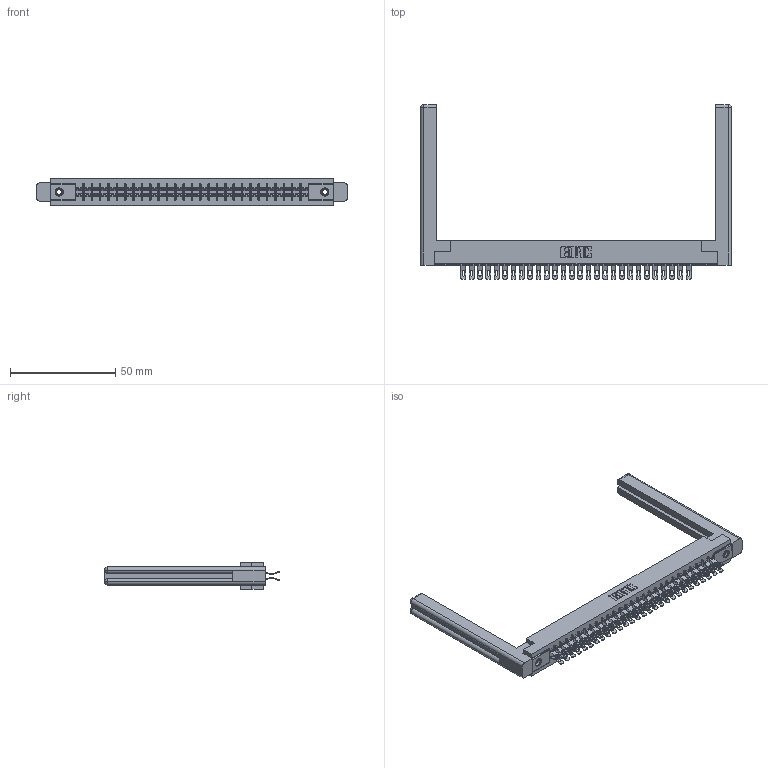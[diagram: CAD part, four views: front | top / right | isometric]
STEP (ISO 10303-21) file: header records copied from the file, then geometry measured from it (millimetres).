
FILE_DESCRIPTION (( 'STEP AP203' ), '1' );
FILE_NAME ('305-056-555-558.STEP', '2019-09-09T23:57:06', ( '' ), ( '' ), 'SwSTEP 2.0', 'SolidWorks 2016', '' );
FILE_SCHEMA (( 'CONFIG_CONTROL_DESIGN' ));
Length unit declared in the file: inch
Products named in the file (5): 305-056-555-558; 307-220-058; 305-290-001_555; 345-250-001_345-250-001-102; 305 Part_.156 Dia
Assembly tree (61 placements, depth 2):
  305-056-555-558
    305 Part_.156 Dia
    305-290-001_555  x56
    345-250-001_345-250-001-102  x2
    307-220-058  x2
Bounding box: 147.57 x 83.06 x 12.7 mm (x, y, z)
Volume: 22245.3 mm3; surface area: 25410.8 mm2
Topology: 61 solids, 61 shells, 3954 faces, 11730 edges, 7656 vertices
Faces by surface type: plane 1944, cylinder 1874, sphere 112, cone 12, torus 12
Entity records: 35278 total; most frequent: CARTESIAN_POINT 5871, ORIENTED_EDGE 5758, DIRECTION 5647, EDGE_CURVE 2879, LINE 2283, VECTOR 2283, VERTEX_POINT 1836, AXIS2_PLACEMENT_3D 1682
